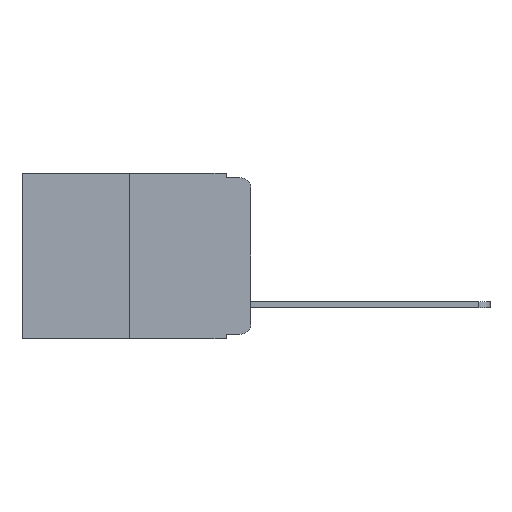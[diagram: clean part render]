
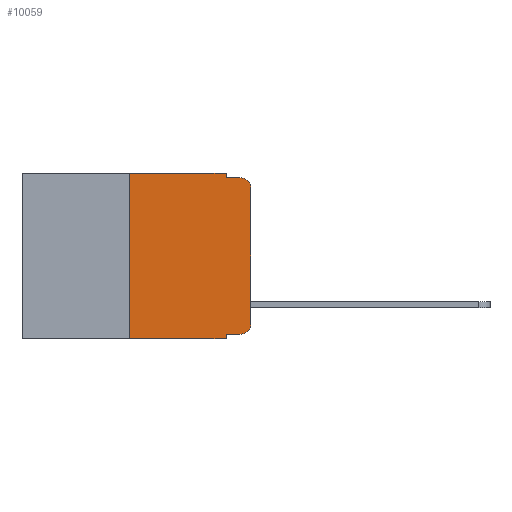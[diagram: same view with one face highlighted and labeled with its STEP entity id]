
A CAD part, left-side view. The second image highlights one B-rep face of the part: STEP entity #10059.
In plain terms, the highlighted planar face has unit normal (-1, 0, 0).
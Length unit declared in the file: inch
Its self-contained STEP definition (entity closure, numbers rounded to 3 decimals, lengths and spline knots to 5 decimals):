
#219 = CIRCLE ( 'NONE', #8693, 0.02 ) ;
#306 = CIRCLE ( 'NONE', #10979, 0.02 ) ;
#307 = LINE ( 'NONE', #10875, #15900 ) ;
#649 = EDGE_CURVE ( 'NONE', #11803, #10108, #7665, .T. ) ;
#838 = CARTESIAN_POINT ( 'NONE',  ( 0., 0.02, -0.313 ) ) ;
#1073 = CARTESIAN_POINT ( 'NONE',  ( 0., 0.25, 0. ) ) ;
#1499 = VECTOR ( 'NONE', #15177, 39.37008 ) ;
#1564 = DIRECTION ( 'NONE',  ( 0., -1., 0. ) ) ;
#1597 = CARTESIAN_POINT ( 'NONE',  ( 0., 0.473, -0.343 ) ) ;
#1841 = DIRECTION ( 'NONE',  ( 0., 0., -1. ) ) ;
#2023 = CARTESIAN_POINT ( 'NONE',  ( 0., 0.02, -0.333 ) ) ;
#2289 = VECTOR ( 'NONE', #18956, 39.37008 ) ;
#2362 = ORIENTED_EDGE ( 'NONE', *, *, #13121, .F. ) ;
#2463 = ORIENTED_EDGE ( 'NONE', *, *, #11873, .T. ) ;
#2575 = LINE ( 'NONE', #9080, #19324 ) ;
#2841 = CARTESIAN_POINT ( 'NONE',  ( 0., 0.02, -0.01 ) ) ;
#3198 = DIRECTION ( 'NONE',  ( -1., 0., 0. ) ) ;
#3834 = CARTESIAN_POINT ( 'NONE',  ( 0., 0.051, 0. ) ) ;
#4622 = CARTESIAN_POINT ( 'NONE',  ( 0., 0.25, 0. ) ) ;
#5014 = EDGE_CURVE ( 'NONE', #16534, #8674, #2575, .T. ) ;
#5467 = EDGE_CURVE ( 'NONE', #10108, #13560, #306, .T. ) ;
#5527 = CARTESIAN_POINT ( 'NONE',  ( 0., 0.25, -0.343 ) ) ;
#6010 = ORIENTED_EDGE ( 'NONE', *, *, #649, .T. ) ;
#6016 = VERTEX_POINT ( 'NONE', #14896 ) ;
#6045 = LINE ( 'NONE', #1597, #15497 ) ;
#6266 = FACE_OUTER_BOUND ( 'NONE', #12037, .T. ) ;
#6719 = DIRECTION ( 'NONE',  ( 0., -1., 0. ) ) ;
#7412 = VERTEX_POINT ( 'NONE', #5527 ) ;
#7570 = CARTESIAN_POINT ( 'NONE',  ( 0., 0.473, 0. ) ) ;
#7665 = LINE ( 'NONE', #17174, #9081 ) ;
#7672 = VERTEX_POINT ( 'NONE', #10583 ) ;
#7759 = DIRECTION ( 'NONE',  ( 0., 0., -1. ) ) ;
#8674 = VERTEX_POINT ( 'NONE', #2841 ) ;
#8693 = AXIS2_PLACEMENT_3D ( 'NONE', #12232, #3198, #1841 ) ;
#8750 = CARTESIAN_POINT ( 'NONE',  ( 0., 0., -0.03 ) ) ;
#8881 = ORIENTED_EDGE ( 'NONE', *, *, #9258, .T. ) ;
#9017 = DIRECTION ( 'NONE',  ( 0., 0., -1. ) ) ;
#9080 = CARTESIAN_POINT ( 'NONE',  ( 0., 0.051, -0.01 ) ) ;
#9081 = VECTOR ( 'NONE', #6719, 39.37008 ) ;
#9258 = EDGE_CURVE ( 'NONE', #7412, #6016, #6045, .T. ) ;
#9283 = CARTESIAN_POINT ( 'NONE',  ( 0., 0.051, -0.333 ) ) ;
#10059 = ADVANCED_FACE ( 'NONE', ( #6266 ), #18027, .F. ) ;
#10108 = VERTEX_POINT ( 'NONE', #2023 ) ;
#10111 = CARTESIAN_POINT ( 'NONE',  ( 0., 0., 0. ) ) ;
#10558 = CARTESIAN_POINT ( 'NONE',  ( 0., 0.051, 0. ) ) ;
#10566 = VECTOR ( 'NONE', #19529, 39.37008 ) ;
#10583 = CARTESIAN_POINT ( 'NONE',  ( 0., 0.051, 0. ) ) ;
#10818 = EDGE_CURVE ( 'NONE', #19126, #7672, #307, .T. ) ;
#10875 = CARTESIAN_POINT ( 'NONE',  ( 0., 0.473, 0. ) ) ;
#10979 = AXIS2_PLACEMENT_3D ( 'NONE', #838, #19231, #7759 ) ;
#11443 = ORIENTED_EDGE ( 'NONE', *, *, #16271, .T. ) ;
#11732 = ORIENTED_EDGE ( 'NONE', *, *, #10818, .F. ) ;
#11803 = VERTEX_POINT ( 'NONE', #9283 ) ;
#11864 = DIRECTION ( 'NONE',  ( 0., -1., 0. ) ) ;
#11873 = EDGE_CURVE ( 'NONE', #14109, #8674, #219, .T. ) ;
#12037 = EDGE_LOOP ( 'NONE', ( #11443, #2463, #13000, #17599, #11732, #15396, #8881, #2362, #6010, #12539 ) ) ;
#12232 = CARTESIAN_POINT ( 'NONE',  ( 0., 0.02, -0.03 ) ) ;
#12539 = ORIENTED_EDGE ( 'NONE', *, *, #5467, .T. ) ;
#12795 = CARTESIAN_POINT ( 'NONE',  ( 0., 0.051, -0.01 ) ) ;
#13000 = ORIENTED_EDGE ( 'NONE', *, *, #5014, .F. ) ;
#13121 = EDGE_CURVE ( 'NONE', #11803, #6016, #17168, .T. ) ;
#13560 = VERTEX_POINT ( 'NONE', #15157 ) ;
#13758 = LINE ( 'NONE', #4622, #1499 ) ;
#13971 = DIRECTION ( 'NONE',  ( 0., -1., 0. ) ) ;
#14109 = VERTEX_POINT ( 'NONE', #8750 ) ;
#14652 = EDGE_CURVE ( 'NONE', #7672, #16534, #16447, .T. ) ;
#14896 = CARTESIAN_POINT ( 'NONE',  ( 0., 0.051, -0.343 ) ) ;
#15157 = CARTESIAN_POINT ( 'NONE',  ( 0., 0., -0.313 ) ) ;
#15177 = DIRECTION ( 'NONE',  ( 0., 0., 1. ) ) ;
#15209 = DIRECTION ( 'NONE',  ( 1., 0., 0. ) ) ;
#15362 = AXIS2_PLACEMENT_3D ( 'NONE', #7570, #15209, #9017 ) ;
#15396 = ORIENTED_EDGE ( 'NONE', *, *, #19468, .F. ) ;
#15497 = VECTOR ( 'NONE', #11864, 39.37008 ) ;
#15900 = VECTOR ( 'NONE', #13971, 39.37008 ) ;
#16271 = EDGE_CURVE ( 'NONE', #13560, #14109, #17528, .T. ) ;
#16447 = LINE ( 'NONE', #3834, #2289 ) ;
#16534 = VERTEX_POINT ( 'NONE', #12795 ) ;
#17168 = LINE ( 'NONE', #10558, #10566 ) ;
#17174 = CARTESIAN_POINT ( 'NONE',  ( 0., 0.051, -0.333 ) ) ;
#17528 = LINE ( 'NONE', #10111, #18969 ) ;
#17599 = ORIENTED_EDGE ( 'NONE', *, *, #14652, .F. ) ;
#18001 = DIRECTION ( 'NONE',  ( 0., 0., 1. ) ) ;
#18027 = PLANE ( 'NONE',  #15362 ) ;
#18956 = DIRECTION ( 'NONE',  ( 0., 0., -1. ) ) ;
#18969 = VECTOR ( 'NONE', #18001, 39.37008 ) ;
#19126 = VERTEX_POINT ( 'NONE', #1073 ) ;
#19231 = DIRECTION ( 'NONE',  ( -1., 0., 0. ) ) ;
#19324 = VECTOR ( 'NONE', #1564, 39.37008 ) ;
#19468 = EDGE_CURVE ( 'NONE', #7412, #19126, #13758, .T. ) ;
#19529 = DIRECTION ( 'NONE',  ( 0., 0., -1. ) ) ;
